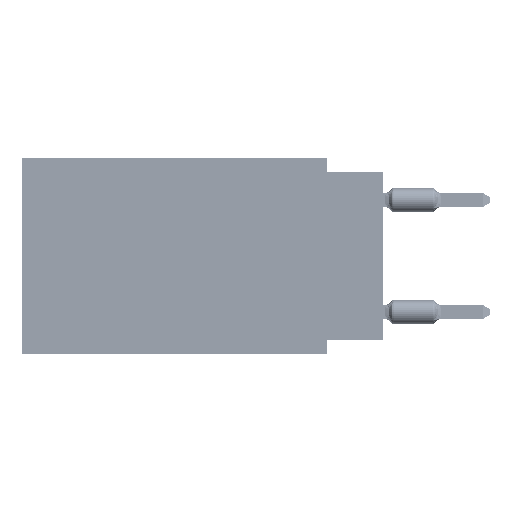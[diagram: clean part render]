
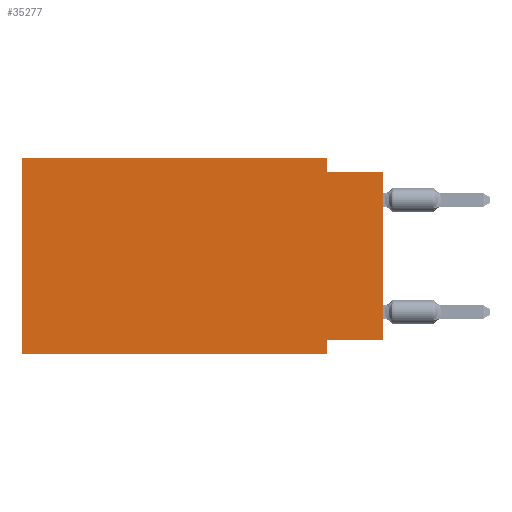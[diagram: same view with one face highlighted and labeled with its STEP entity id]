
A CAD part, left-side view. The second image highlights one B-rep face of the part: STEP entity #35277.
In plain terms, the highlighted planar face has unit normal (-1, 0, 0).
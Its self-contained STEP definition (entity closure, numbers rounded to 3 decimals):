
#2056 = EDGE_CURVE ( 'NONE', #34151, #12818, #76672, .T. ) ;
#2531 = EDGE_CURVE ( 'NONE', #66442, #91105, #61534, .T. ) ;
#3026 = DIRECTION ( 'NONE',  ( 0., 1., 0. ) ) ;
#3817 = CARTESIAN_POINT ( 'NONE',  ( 0., 2.54, -8.89 ) ) ;
#5894 = FACE_OUTER_BOUND ( 'NONE', #40956, .T. ) ;
#8384 = DIRECTION ( 'NONE',  ( 0., -1., 0. ) ) ;
#9887 = VERTEX_POINT ( 'NONE', #50299 ) ;
#11918 = DIRECTION ( 'NONE',  ( 0., -1., 0. ) ) ;
#12040 = CARTESIAN_POINT ( 'NONE',  ( 0., 2.54, 0. ) ) ;
#12500 = LINE ( 'NONE', #26073, #69046 ) ;
#12818 = VERTEX_POINT ( 'NONE', #74487 ) ;
#15790 = VECTOR ( 'NONE', #11918, 1000. ) ;
#16952 = CARTESIAN_POINT ( 'NONE',  ( 0., 2.54, 0. ) ) ;
#17847 = ORIENTED_EDGE ( 'NONE', *, *, #2531, .F. ) ;
#18999 = DIRECTION ( 'NONE',  ( 1., 0., 0. ) ) ;
#20195 = CARTESIAN_POINT ( 'NONE',  ( 0., 16.383, -8.89 ) ) ;
#20801 = ORIENTED_EDGE ( 'NONE', *, *, #23456, .F. ) ;
#23454 = CARTESIAN_POINT ( 'NONE',  ( 0., 0., -0.635 ) ) ;
#23456 = EDGE_CURVE ( 'NONE', #12818, #48335, #31989, .T. ) ;
#25541 = DIRECTION ( 'NONE',  ( 0., 0., 1. ) ) ;
#26073 = CARTESIAN_POINT ( 'NONE',  ( 0., 0., 0. ) ) ;
#26527 = LINE ( 'NONE', #20195, #63584 ) ;
#31989 = LINE ( 'NONE', #90177, #69825 ) ;
#32244 = ORIENTED_EDGE ( 'NONE', *, *, #34396, .F. ) ;
#32328 = CARTESIAN_POINT ( 'NONE',  ( 0., 16.383, 0. ) ) ;
#33240 = LINE ( 'NONE', #40510, #15790 ) ;
#33994 = CARTESIAN_POINT ( 'NONE',  ( 0., 0., -8.255 ) ) ;
#34151 = VERTEX_POINT ( 'NONE', #33994 ) ;
#34396 = EDGE_CURVE ( 'NONE', #9887, #50022, #84180, .T. ) ;
#35168 = AXIS2_PLACEMENT_3D ( 'NONE', #50442, #18999, #35426 ) ;
#35277 = ADVANCED_FACE ( 'NONE', ( #5894 ), #78117, .F. ) ;
#35426 = DIRECTION ( 'NONE',  ( 0., 0., -1. ) ) ;
#36487 = CARTESIAN_POINT ( 'NONE',  ( 0., 16.383, 0. ) ) ;
#39411 = EDGE_CURVE ( 'NONE', #91105, #78959, #33240, .T. ) ;
#40510 = CARTESIAN_POINT ( 'NONE',  ( 0., 0., -0.635 ) ) ;
#40580 = DIRECTION ( 'NONE',  ( 0., -1., 0. ) ) ;
#40956 = EDGE_LOOP ( 'NONE', ( #62021, #60144, #17847, #49160, #32244, #78360, #20801, #59157 ) ) ;
#42893 = VECTOR ( 'NONE', #76545, 1000. ) ;
#47437 = VECTOR ( 'NONE', #25541, 1000. ) ;
#48335 = VERTEX_POINT ( 'NONE', #3817 ) ;
#48360 = DIRECTION ( 'NONE',  ( 0., 0., 1. ) ) ;
#49160 = ORIENTED_EDGE ( 'NONE', *, *, #86911, .F. ) ;
#50022 = VERTEX_POINT ( 'NONE', #78643 ) ;
#50299 = CARTESIAN_POINT ( 'NONE',  ( 0., 16.383, -8.89 ) ) ;
#50442 = CARTESIAN_POINT ( 'NONE',  ( 0., 16.383, 0. ) ) ;
#55360 = CARTESIAN_POINT ( 'NONE',  ( 0., 2.54, -0.635 ) ) ;
#59157 = ORIENTED_EDGE ( 'NONE', *, *, #2056, .F. ) ;
#60144 = ORIENTED_EDGE ( 'NONE', *, *, #39411, .F. ) ;
#61534 = LINE ( 'NONE', #16952, #42893 ) ;
#61553 = DIRECTION ( 'NONE',  ( 0., 0., -1. ) ) ;
#62021 = ORIENTED_EDGE ( 'NONE', *, *, #65832, .T. ) ;
#63584 = VECTOR ( 'NONE', #40580, 1000. ) ;
#65832 = EDGE_CURVE ( 'NONE', #34151, #78959, #12500, .T. ) ;
#66442 = VERTEX_POINT ( 'NONE', #12040 ) ;
#69046 = VECTOR ( 'NONE', #48360, 1000. ) ;
#69825 = VECTOR ( 'NONE', #61553, 1000. ) ;
#73324 = LINE ( 'NONE', #36487, #81852 ) ;
#74487 = CARTESIAN_POINT ( 'NONE',  ( 0., 2.54, -8.255 ) ) ;
#76195 = CARTESIAN_POINT ( 'NONE',  ( 0., 0., -8.255 ) ) ;
#76545 = DIRECTION ( 'NONE',  ( 0., 0., -1. ) ) ;
#76672 = LINE ( 'NONE', #76195, #78393 ) ;
#78117 = PLANE ( 'NONE',  #35168 ) ;
#78360 = ORIENTED_EDGE ( 'NONE', *, *, #89247, .T. ) ;
#78393 = VECTOR ( 'NONE', #3026, 1000. ) ;
#78643 = CARTESIAN_POINT ( 'NONE',  ( 0., 16.383, 0. ) ) ;
#78959 = VERTEX_POINT ( 'NONE', #23454 ) ;
#81852 = VECTOR ( 'NONE', #8384, 1000. ) ;
#84180 = LINE ( 'NONE', #32328, #47437 ) ;
#86911 = EDGE_CURVE ( 'NONE', #50022, #66442, #73324, .T. ) ;
#89247 = EDGE_CURVE ( 'NONE', #9887, #48335, #26527, .T. ) ;
#90177 = CARTESIAN_POINT ( 'NONE',  ( 0., 2.54, -8.89 ) ) ;
#91105 = VERTEX_POINT ( 'NONE', #55360 ) ;
